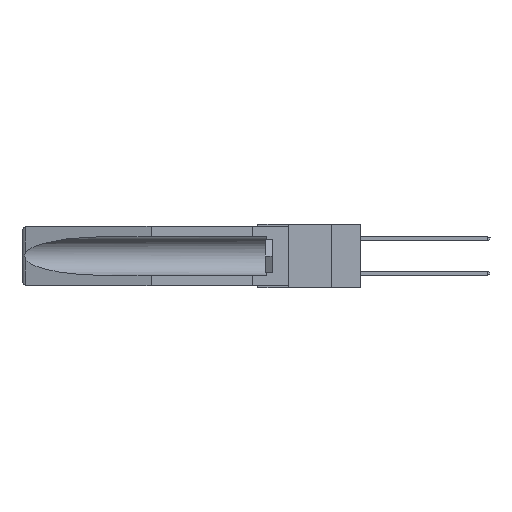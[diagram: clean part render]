
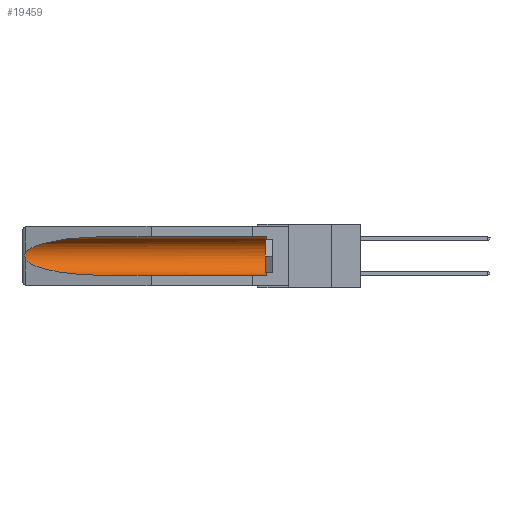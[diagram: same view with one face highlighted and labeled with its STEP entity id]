
A CAD part, left-side view. The second image highlights one B-rep face of the part: STEP entity #19459.
In plain terms, the highlighted cylindrical face has radius 2.857 mm (diameter 5.715 mm), a partial arc.
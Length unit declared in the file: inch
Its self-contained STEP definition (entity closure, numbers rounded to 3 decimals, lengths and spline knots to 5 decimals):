
#362 = CARTESIAN_POINT ( 'NONE',  ( 0.25451, 1.48313, -0.09465 ) ) ;
#376 = EDGE_CURVE ( 'NONE', #28078, #5852, #11832, .T. ) ;
#609 = FACE_OUTER_BOUND ( 'NONE', #27707, .T. ) ;
#1786 = CARTESIAN_POINT ( 'NONE',  ( 0.26537, 1.52718, -0.19328 ) ) ;
#2051 = CARTESIAN_POINT ( 'NONE',  ( 0.26537, 1.52718, -0.19328 ) ) ;
#2301 = DIRECTION ( 'NONE',  ( 0., 1., 0. ) ) ;
#2418 = EDGE_CURVE ( 'NONE', #24379, #24159, #20371, .T. ) ;
#3595 = ORIENTED_EDGE ( 'NONE', *, *, #2418, .T. ) ;
#4612 = DIRECTION ( 'NONE',  ( 0., 0., 1. ) ) ;
#5064 = CIRCLE ( 'NONE', #24221, 0.1125 ) ;
#5668 = ORIENTED_EDGE ( 'NONE', *, *, #13948, .T. ) ;
#5852 = VERTEX_POINT ( 'NONE', #23132 ) ;
#5985 = CARTESIAN_POINT ( 'NONE',  ( 0.21114, 1.30732, -0.284 ) ) ;
#6217 = DIRECTION ( 'NONE',  ( 0., 1., 0. ) ) ;
#6324 = CARTESIAN_POINT ( 'NONE',  ( 0.2675, 1.53308, -0.16763 ) ) ;
#6734 = CYLINDRICAL_SURFACE ( 'NONE', #11112, 0.1125 ) ;
#8313 = CARTESIAN_POINT ( 'NONE',  ( 0.26597, 1.52961, -0.15275 ) ) ;
#8506 = CARTESIAN_POINT ( 'NONE',  ( 0.2675, 1.53308, -0.17534 ) ) ;
#8610 = CARTESIAN_POINT ( 'NONE',  ( 0.2673, 1.5327, -0.16383 ) ) ;
#8641 = CARTESIAN_POINT ( 'NONE',  ( 0.155, 1.07973, -0.284 ) ) ;
#9113 = CARTESIAN_POINT ( 'NONE',  ( 0.26537, 1.52718, -0.14972 ) ) ;
#10354 = ORIENTED_EDGE ( 'NONE', *, *, #376, .T. ) ;
#10853 = EDGE_CURVE ( 'NONE', #18688, #24379, #5064, .T. ) ;
#10910 = VECTOR ( 'NONE', #15107, 39.37008 ) ;
#10950 = CARTESIAN_POINT ( 'NONE',  ( 0.26537, 1.52718, -0.14972 ) ) ;
#11112 = AXIS2_PLACEMENT_3D ( 'NONE', #17040, #6217, #25433 ) ;
#11619 = ORIENTED_EDGE ( 'NONE', *, *, #10853, .T. ) ;
#11832 =( BOUNDED_CURVE ( )  B_SPLINE_CURVE ( 3, ( #1786, #17087, #5985, #8641 ),
 .UNSPECIFIED., .F., .F. ) 
 B_SPLINE_CURVE_WITH_KNOTS ( ( 4, 4 ),
 ( 0.1948, 1.5708 ),
 .UNSPECIFIED. ) 
 CURVE ( )  GEOMETRIC_REPRESENTATION_ITEM ( )  RATIONAL_B_SPLINE_CURVE ( ( 1., 0.848, 0.848, 1. ) ) 
 REPRESENTATION_ITEM ( '' )  );
#12775 = CARTESIAN_POINT ( 'NONE',  ( 0.26654, 1.53092, -0.15636 ) ) ;
#13120 = CARTESIAN_POINT ( 'NONE',  ( 0.155, 0.126, -0.1715 ) ) ;
#13374 = CARTESIAN_POINT ( 'NONE',  ( 0.21114, 1.30732, -0.059 ) ) ;
#13506 = CARTESIAN_POINT ( 'NONE',  ( 0.155, 0.126, -0.284 ) ) ;
#13948 = EDGE_CURVE ( 'NONE', #19625, #28078, #22747, .T. ) ;
#14352 = ORIENTED_EDGE ( 'NONE', *, *, #25411, .F. ) ;
#14403 = CARTESIAN_POINT ( 'NONE',  ( 0.155, 1.07973, -0.059 ) ) ;
#14523 = LINE ( 'NONE', #23904, #21986 ) ;
#15078 = CARTESIAN_POINT ( 'NONE',  ( 0.26655, 1.53094, -0.18657 ) ) ;
#15107 = DIRECTION ( 'NONE',  ( 0., 1., 0. ) ) ;
#15686 = ORIENTED_EDGE ( 'NONE', *, *, #20377, .T. ) ;
#17040 = CARTESIAN_POINT ( 'NONE',  ( 0.155, -0.30754, -0.1715 ) ) ;
#17087 = CARTESIAN_POINT ( 'NONE',  ( 0.25451, 1.48313, -0.24835 ) ) ;
#17768 =( BOUNDED_CURVE ( )  B_SPLINE_CURVE ( 3, ( #18129, #13374, #362, #9113 ),
 .UNSPECIFIED., .F., .F. ) 
 B_SPLINE_CURVE_WITH_KNOTS ( ( 4, 4 ),
 ( 4.71239, 6.08839 ),
 .UNSPECIFIED. ) 
 CURVE ( )  GEOMETRIC_REPRESENTATION_ITEM ( )  RATIONAL_B_SPLINE_CURVE ( ( 1., 0.848, 0.848, 1. ) ) 
 REPRESENTATION_ITEM ( '' )  );
#18129 = CARTESIAN_POINT ( 'NONE',  ( 0.155, 1.07973, -0.059 ) ) ;
#18688 = VERTEX_POINT ( 'NONE', #13506 ) ;
#18700 = CARTESIAN_POINT ( 'NONE',  ( 0.155, 0.126, -0.059 ) ) ;
#19134 = CARTESIAN_POINT ( 'NONE',  ( 0.26537, 1.52718, -0.14972 ) ) ;
#19252 = CARTESIAN_POINT ( 'NONE',  ( 0.155, -0.30754, -0.059 ) ) ;
#19459 = ADVANCED_FACE ( 'NONE', ( #609 ), #6734, .F. ) ;
#19625 = VERTEX_POINT ( 'NONE', #10950 ) ;
#19857 = DIRECTION ( 'NONE',  ( 0., -1., 0. ) ) ;
#20371 = LINE ( 'NONE', #19252, #10910 ) ;
#20377 = EDGE_CURVE ( 'NONE', #24159, #19625, #17768, .T. ) ;
#21986 = VECTOR ( 'NONE', #2301, 39.37008 ) ;
#22747 = B_SPLINE_CURVE_WITH_KNOTS ( 'NONE', 3,
 ( #19134, #8313, #12775, #8610, #6324, #8506, #23639, #15078, #25910, #2051 ),
 .UNSPECIFIED., .F., .F.,
 ( 4, 2, 2, 2, 4 ),
 ( 0., 0.00029, 0.00058, 0.00087, 0.00117 ),
 .UNSPECIFIED. ) ;
#23110 = CARTESIAN_POINT ( 'NONE',  ( 0.26537, 1.52718, -0.19328 ) ) ;
#23132 = CARTESIAN_POINT ( 'NONE',  ( 0.155, 1.07973, -0.284 ) ) ;
#23639 = CARTESIAN_POINT ( 'NONE',  ( 0.2673, 1.53269, -0.17917 ) ) ;
#23904 = CARTESIAN_POINT ( 'NONE',  ( 0.155, -0.30754, -0.284 ) ) ;
#24159 = VERTEX_POINT ( 'NONE', #14403 ) ;
#24221 = AXIS2_PLACEMENT_3D ( 'NONE', #13120, #19857, #4612 ) ;
#24379 = VERTEX_POINT ( 'NONE', #18700 ) ;
#25411 = EDGE_CURVE ( 'NONE', #18688, #5852, #14523, .T. ) ;
#25433 = DIRECTION ( 'NONE',  ( 0., 0., 1. ) ) ;
#25910 = CARTESIAN_POINT ( 'NONE',  ( 0.26597, 1.5296, -0.19026 ) ) ;
#27707 = EDGE_LOOP ( 'NONE', ( #15686, #5668, #10354, #14352, #11619, #3595 ) ) ;
#28078 = VERTEX_POINT ( 'NONE', #23110 ) ;
